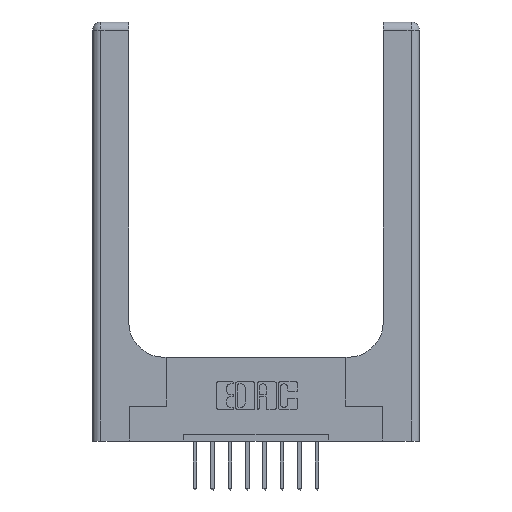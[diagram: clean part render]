
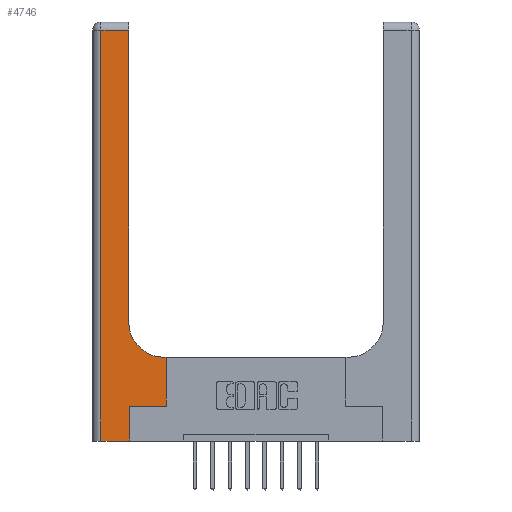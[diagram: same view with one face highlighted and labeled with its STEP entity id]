
A CAD part, top view. The second image highlights one B-rep face of the part: STEP entity #4746.
In plain terms, the highlighted planar face has unit normal (0, 0, 1).
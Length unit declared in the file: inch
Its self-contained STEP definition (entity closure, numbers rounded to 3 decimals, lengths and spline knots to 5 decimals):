
#291 = DIRECTION ( 'NONE',  ( 1., 0., 0. ) ) ;
#409 = DIRECTION ( 'NONE',  ( 0., 0., -1. ) ) ;
#646 = VECTOR ( 'NONE', #291, 39.37008 ) ;
#677 = CARTESIAN_POINT ( 'NONE',  ( 0., 2.94, 0.37 ) ) ;
#710 = EDGE_CURVE ( 'NONE', #9828, #5711, #3974, .T. ) ;
#834 = VERTEX_POINT ( 'NONE', #13818 ) ;
#923 = FACE_OUTER_BOUND ( 'NONE', #9296, .T. ) ;
#934 = ORIENTED_EDGE ( 'NONE', *, *, #1130, .T. ) ;
#993 = DIRECTION ( 'NONE',  ( 0., 0., -1. ) ) ;
#1092 = EDGE_CURVE ( 'NONE', #6768, #9828, #9956, .T. ) ;
#1130 = EDGE_CURVE ( 'NONE', #6052, #834, #12431, .T. ) ;
#1226 = LINE ( 'NONE', #8265, #2026 ) ;
#1440 = CARTESIAN_POINT ( 'NONE',  ( 0.265, 0.25, 0.37 ) ) ;
#1472 = CARTESIAN_POINT ( 'NONE',  ( 0.528, 0.25, 0.37 ) ) ;
#1839 = CARTESIAN_POINT ( 'NONE',  ( 0., 0., 0.37 ) ) ;
#1956 = VERTEX_POINT ( 'NONE', #5150 ) ;
#2026 = VECTOR ( 'NONE', #4401, 39.37008 ) ;
#2174 = VERTEX_POINT ( 'NONE', #9824 ) ;
#2593 = VECTOR ( 'NONE', #4109, 39.37008 ) ;
#2691 = CARTESIAN_POINT ( 'NONE',  ( 0.265, 0., 0.37 ) ) ;
#3061 = DIRECTION ( 'NONE',  ( 1., 0., 0. ) ) ;
#3148 = VECTOR ( 'NONE', #15111, 39.37008 ) ;
#3358 = DIRECTION ( 'NONE',  ( -1., 0., 0. ) ) ;
#3653 = EDGE_CURVE ( 'NONE', #5711, #2174, #1226, .T. ) ;
#3956 = DIRECTION ( 'NONE',  ( 0., -1., 0. ) ) ;
#3974 = LINE ( 'NONE', #1839, #10186 ) ;
#4095 = VECTOR ( 'NONE', #4134, 39.37008 ) ;
#4109 = DIRECTION ( 'NONE',  ( 0., 1., 0. ) ) ;
#4134 = DIRECTION ( 'NONE',  ( 0., 1., 0. ) ) ;
#4401 = DIRECTION ( 'NONE',  ( 0., 1., 0. ) ) ;
#4585 = CARTESIAN_POINT ( 'NONE',  ( 0.06, 0., 0.37 ) ) ;
#4746 = ADVANCED_FACE ( 'NONE', ( #923 ), #6814, .F. ) ;
#4995 = CARTESIAN_POINT ( 'NONE',  ( 0.51, 0.85, 0.37 ) ) ;
#5150 = CARTESIAN_POINT ( 'NONE',  ( 0.26, 0.85, 0.37 ) ) ;
#5289 = EDGE_CURVE ( 'NONE', #7019, #1956, #12130, .T. ) ;
#5445 = CARTESIAN_POINT ( 'NONE',  ( 0.26, 3., 0.37 ) ) ;
#5711 = VERTEX_POINT ( 'NONE', #2691 ) ;
#5790 = ORIENTED_EDGE ( 'NONE', *, *, #8674, .T. ) ;
#6052 = VERTEX_POINT ( 'NONE', #1472 ) ;
#6336 = CARTESIAN_POINT ( 'NONE',  ( 0.06, 3., 0.37 ) ) ;
#6382 = EDGE_CURVE ( 'NONE', #2174, #6052, #11980, .T. ) ;
#6768 = VERTEX_POINT ( 'NONE', #8774 ) ;
#6814 = PLANE ( 'NONE',  #6926 ) ;
#6887 = ORIENTED_EDGE ( 'NONE', *, *, #6382, .T. ) ;
#6926 = AXIS2_PLACEMENT_3D ( 'NONE', #11524, #993, #3358 ) ;
#7019 = VERTEX_POINT ( 'NONE', #14160 ) ;
#7809 = ORIENTED_EDGE ( 'NONE', *, *, #710, .T. ) ;
#7833 = EDGE_CURVE ( 'NONE', #1956, #12732, #8809, .T. ) ;
#8254 = CARTESIAN_POINT ( 'NONE',  ( 0.26, 0.6, 0.37 ) ) ;
#8265 = CARTESIAN_POINT ( 'NONE',  ( 0.265, 0., 0.37 ) ) ;
#8674 = EDGE_CURVE ( 'NONE', #834, #7019, #9422, .T. ) ;
#8774 = CARTESIAN_POINT ( 'NONE',  ( 0.06, 2.94, 0.37 ) ) ;
#8809 = LINE ( 'NONE', #5445, #4095 ) ;
#8819 = ORIENTED_EDGE ( 'NONE', *, *, #9032, .T. ) ;
#8870 = DIRECTION ( 'NONE',  ( -1., 0., 0. ) ) ;
#8998 = ORIENTED_EDGE ( 'NONE', *, *, #3653, .T. ) ;
#9032 = EDGE_CURVE ( 'NONE', #12732, #6768, #11209, .T. ) ;
#9296 = EDGE_LOOP ( 'NONE', ( #9901, #8819, #12620, #7809, #8998, #6887, #934, #5790, #14719 ) ) ;
#9422 = LINE ( 'NONE', #8254, #3148 ) ;
#9824 = CARTESIAN_POINT ( 'NONE',  ( 0.265, 0.25, 0.37 ) ) ;
#9828 = VERTEX_POINT ( 'NONE', #4585 ) ;
#9901 = ORIENTED_EDGE ( 'NONE', *, *, #7833, .T. ) ;
#9956 = LINE ( 'NONE', #6336, #14127 ) ;
#10186 = VECTOR ( 'NONE', #3061, 39.37008 ) ;
#10861 = DIRECTION ( 'NONE',  ( 1., 0., 0. ) ) ;
#11209 = LINE ( 'NONE', #677, #14194 ) ;
#11524 = CARTESIAN_POINT ( 'NONE',  ( 0., 3., 0.37 ) ) ;
#11980 = LINE ( 'NONE', #1440, #646 ) ;
#12130 = CIRCLE ( 'NONE', #14818, 0.25 ) ;
#12431 = LINE ( 'NONE', #13423, #2593 ) ;
#12555 = CARTESIAN_POINT ( 'NONE',  ( 0.26, 2.94, 0.37 ) ) ;
#12620 = ORIENTED_EDGE ( 'NONE', *, *, #1092, .T. ) ;
#12732 = VERTEX_POINT ( 'NONE', #12555 ) ;
#13423 = CARTESIAN_POINT ( 'NONE',  ( 0.528, 0.25, 0.37 ) ) ;
#13818 = CARTESIAN_POINT ( 'NONE',  ( 0.528, 0.6, 0.37 ) ) ;
#14127 = VECTOR ( 'NONE', #3956, 39.37008 ) ;
#14160 = CARTESIAN_POINT ( 'NONE',  ( 0.51, 0.6, 0.37 ) ) ;
#14194 = VECTOR ( 'NONE', #8870, 39.37008 ) ;
#14719 = ORIENTED_EDGE ( 'NONE', *, *, #5289, .T. ) ;
#14818 = AXIS2_PLACEMENT_3D ( 'NONE', #4995, #409, #10861 ) ;
#15111 = DIRECTION ( 'NONE',  ( -1., 0., 0. ) ) ;
